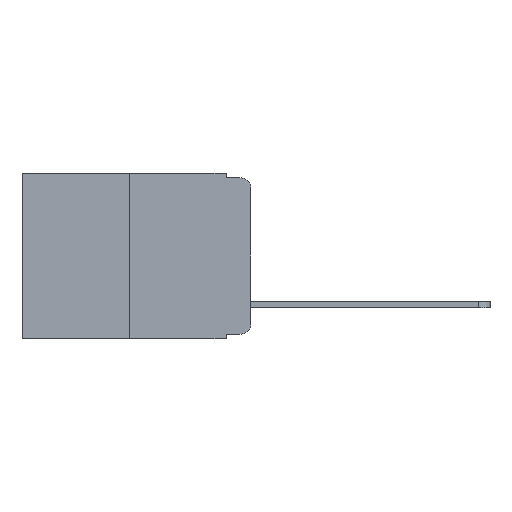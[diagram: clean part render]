
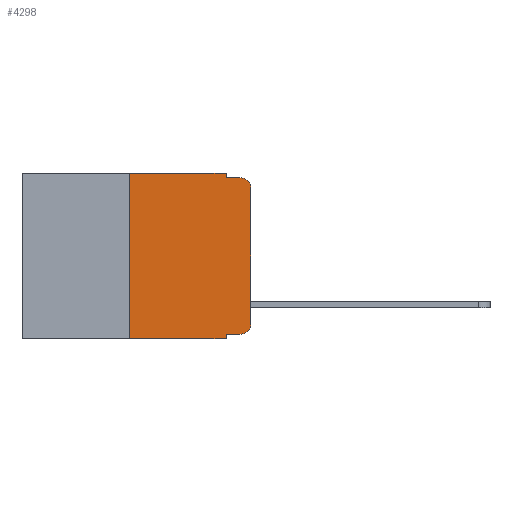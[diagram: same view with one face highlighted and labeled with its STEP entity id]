
A CAD part, left-side view. The second image highlights one B-rep face of the part: STEP entity #4298.
In plain terms, the highlighted planar face has unit normal (-1, 0, 0).
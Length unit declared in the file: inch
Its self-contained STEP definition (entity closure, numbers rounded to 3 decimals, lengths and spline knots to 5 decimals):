
#47 = VERTEX_POINT ( 'NONE', #554 ) ;
#131 = LINE ( 'NONE', #9337, #14935 ) ;
#172 = DIRECTION ( 'NONE',  ( 0., -1., 0. ) ) ;
#201 = FACE_OUTER_BOUND ( 'NONE', #10843, .T. ) ;
#204 = ORIENTED_EDGE ( 'NONE', *, *, #11220, .F. ) ;
#298 = ORIENTED_EDGE ( 'NONE', *, *, #4830, .F. ) ;
#403 = CARTESIAN_POINT ( 'NONE',  ( 0., 0.051, -0.343 ) ) ;
#554 = CARTESIAN_POINT ( 'NONE',  ( 0., 0.051, 0. ) ) ;
#772 = ORIENTED_EDGE ( 'NONE', *, *, #12961, .F. ) ;
#1098 = CARTESIAN_POINT ( 'NONE',  ( 0., 0.051, 0. ) ) ;
#1571 = VERTEX_POINT ( 'NONE', #3618 ) ;
#1959 = ORIENTED_EDGE ( 'NONE', *, *, #15692, .F. ) ;
#2173 = CARTESIAN_POINT ( 'NONE',  ( 0., 0.02, -0.313 ) ) ;
#2198 = DIRECTION ( 'NONE',  ( 0., 0., -1. ) ) ;
#2443 = VERTEX_POINT ( 'NONE', #14802 ) ;
#2468 = VERTEX_POINT ( 'NONE', #15432 ) ;
#2642 = CARTESIAN_POINT ( 'NONE',  ( 0., 0.473, -0.343 ) ) ;
#3284 = EDGE_CURVE ( 'NONE', #2443, #15841, #18222, .T. ) ;
#3509 = VERTEX_POINT ( 'NONE', #10119 ) ;
#3618 = CARTESIAN_POINT ( 'NONE',  ( 0., 0.051, -0.01 ) ) ;
#3807 = DIRECTION ( 'NONE',  ( 0., 0., -1. ) ) ;
#4108 = LINE ( 'NONE', #6109, #8741 ) ;
#4273 = DIRECTION ( 'NONE',  ( 0., 0., -1. ) ) ;
#4298 = ADVANCED_FACE ( 'NONE', ( #201 ), #6568, .F. ) ;
#4595 = ORIENTED_EDGE ( 'NONE', *, *, #5810, .T. ) ;
#4830 = EDGE_CURVE ( 'NONE', #1571, #15438, #4108, .T. ) ;
#4939 = ORIENTED_EDGE ( 'NONE', *, *, #6317, .F. ) ;
#4950 = CARTESIAN_POINT ( 'NONE',  ( 0., 0.02, -0.01 ) ) ;
#5041 = CARTESIAN_POINT ( 'NONE',  ( 0., 0.25, 0. ) ) ;
#5080 = VERTEX_POINT ( 'NONE', #5041 ) ;
#5205 = ORIENTED_EDGE ( 'NONE', *, *, #16833, .T. ) ;
#5810 = EDGE_CURVE ( 'NONE', #11090, #11563, #17074, .T. ) ;
#5946 = DIRECTION ( 'NONE',  ( 0., -1., 0. ) ) ;
#5980 = VECTOR ( 'NONE', #17162, 39.37008 ) ;
#6109 = CARTESIAN_POINT ( 'NONE',  ( 0., 0.051, -0.01 ) ) ;
#6317 = EDGE_CURVE ( 'NONE', #3509, #11563, #14560, .T. ) ;
#6412 = CARTESIAN_POINT ( 'NONE',  ( 0., 0.02, -0.03 ) ) ;
#6568 = PLANE ( 'NONE',  #15935 ) ;
#7661 = VECTOR ( 'NONE', #16425, 39.37008 ) ;
#7723 = CARTESIAN_POINT ( 'NONE',  ( 0., 0.051, -0.333 ) ) ;
#7929 = DIRECTION ( 'NONE',  ( 0., 0., -1. ) ) ;
#8635 = VECTOR ( 'NONE', #4273, 39.37008 ) ;
#8741 = VECTOR ( 'NONE', #5946, 39.37008 ) ;
#8965 = VECTOR ( 'NONE', #15440, 39.37008 ) ;
#9216 = DIRECTION ( 'NONE',  ( 0., 0., 1. ) ) ;
#9337 = CARTESIAN_POINT ( 'NONE',  ( 0., 0.25, 0. ) ) ;
#10119 = CARTESIAN_POINT ( 'NONE',  ( 0., 0.051, -0.333 ) ) ;
#10843 = EDGE_LOOP ( 'NONE', ( #15512, #15757, #298, #1959, #772, #204, #4595, #4939, #5205, #14644 ) ) ;
#10965 = AXIS2_PLACEMENT_3D ( 'NONE', #6412, #16100, #7929 ) ;
#11090 = VERTEX_POINT ( 'NONE', #12346 ) ;
#11220 = EDGE_CURVE ( 'NONE', #11090, #5080, #131, .T. ) ;
#11563 = VERTEX_POINT ( 'NONE', #403 ) ;
#12127 = CARTESIAN_POINT ( 'NONE',  ( 0., 0., -0.03 ) ) ;
#12346 = CARTESIAN_POINT ( 'NONE',  ( 0., 0.25, -0.343 ) ) ;
#12791 = LINE ( 'NONE', #14202, #8965 ) ;
#12800 = DIRECTION ( 'NONE',  ( -1., 0., 0. ) ) ;
#12961 = EDGE_CURVE ( 'NONE', #5080, #47, #12791, .T. ) ;
#13176 = CIRCLE ( 'NONE', #10965, 0.02 ) ;
#13178 = CARTESIAN_POINT ( 'NONE',  ( 0., 0.051, 0. ) ) ;
#13363 = VECTOR ( 'NONE', #172, 39.37008 ) ;
#13708 = EDGE_CURVE ( 'NONE', #15841, #15438, #13176, .T. ) ;
#14025 = AXIS2_PLACEMENT_3D ( 'NONE', #2173, #12800, #3807 ) ;
#14183 = DIRECTION ( 'NONE',  ( 0., 0., -1. ) ) ;
#14202 = CARTESIAN_POINT ( 'NONE',  ( 0., 0.473, 0. ) ) ;
#14204 = VECTOR ( 'NONE', #2198, 39.37008 ) ;
#14476 = CIRCLE ( 'NONE', #14025, 0.02 ) ;
#14560 = LINE ( 'NONE', #1098, #14204 ) ;
#14644 = ORIENTED_EDGE ( 'NONE', *, *, #17889, .T. ) ;
#14802 = CARTESIAN_POINT ( 'NONE',  ( 0., 0., -0.313 ) ) ;
#14897 = CARTESIAN_POINT ( 'NONE',  ( 0., 0., 0. ) ) ;
#14935 = VECTOR ( 'NONE', #9216, 39.37008 ) ;
#15432 = CARTESIAN_POINT ( 'NONE',  ( 0., 0.02, -0.333 ) ) ;
#15438 = VERTEX_POINT ( 'NONE', #4950 ) ;
#15440 = DIRECTION ( 'NONE',  ( 0., -1., 0. ) ) ;
#15512 = ORIENTED_EDGE ( 'NONE', *, *, #3284, .T. ) ;
#15692 = EDGE_CURVE ( 'NONE', #47, #1571, #16254, .T. ) ;
#15757 = ORIENTED_EDGE ( 'NONE', *, *, #13708, .T. ) ;
#15841 = VERTEX_POINT ( 'NONE', #12127 ) ;
#15935 = AXIS2_PLACEMENT_3D ( 'NONE', #17293, #17370, #14183 ) ;
#16100 = DIRECTION ( 'NONE',  ( -1., 0., 0. ) ) ;
#16254 = LINE ( 'NONE', #13178, #8635 ) ;
#16425 = DIRECTION ( 'NONE',  ( 0., 0., 1. ) ) ;
#16833 = EDGE_CURVE ( 'NONE', #3509, #2468, #17368, .T. ) ;
#17074 = LINE ( 'NONE', #2642, #13363 ) ;
#17162 = DIRECTION ( 'NONE',  ( 0., -1., 0. ) ) ;
#17293 = CARTESIAN_POINT ( 'NONE',  ( 0., 0.473, 0. ) ) ;
#17368 = LINE ( 'NONE', #7723, #5980 ) ;
#17370 = DIRECTION ( 'NONE',  ( 1., 0., 0. ) ) ;
#17889 = EDGE_CURVE ( 'NONE', #2468, #2443, #14476, .T. ) ;
#18222 = LINE ( 'NONE', #14897, #7661 ) ;
